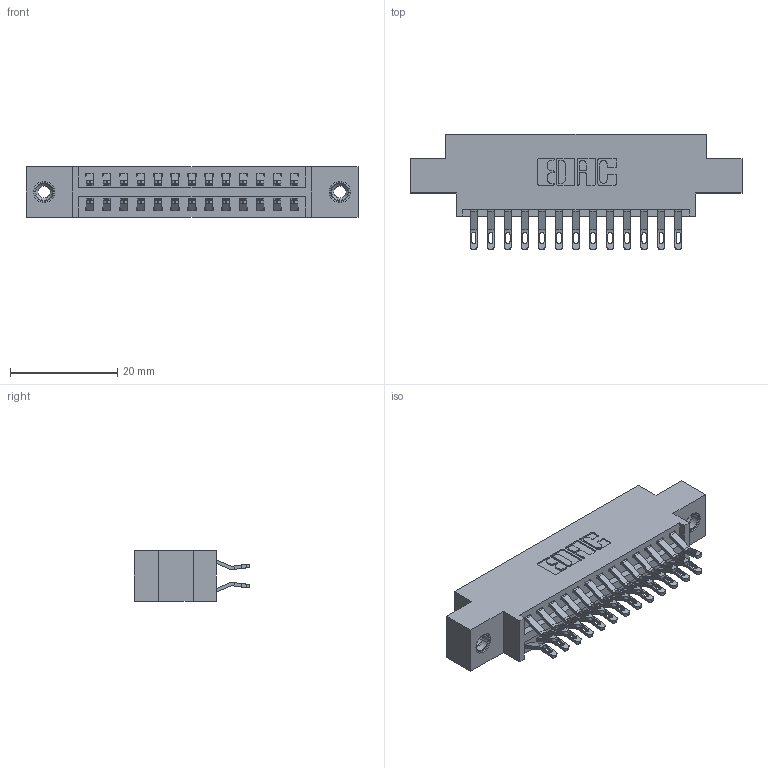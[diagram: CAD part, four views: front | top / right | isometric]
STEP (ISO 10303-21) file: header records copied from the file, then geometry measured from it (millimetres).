
FILE_DESCRIPTION (( 'STEP AP203' ), '1' );
FILE_NAME ('396-026-555-808.STEP', '2018-09-05T00:37:01', ( '' ), ( '' ), 'SwSTEP 2.0', 'SolidWorks 2016', '' );
FILE_SCHEMA (( 'CONFIG_CONTROL_DESIGN' ));
Length unit declared in the file: inch
Products named in the file (4): 346 Part_0.170 Offset - 0.156 Dia-TI; 345-292-001_555 Tail; 345-250-001_345-250-003-102; 396-026-555-808
Assembly tree (29 placements, depth 2):
  396-026-555-808
    346 Part_0.170 Offset - 0.156 Dia-TI
    345-292-001_555 Tail  x26
    345-250-001_345-250-003-102  x2
Bounding box: 61.85 x 21.46 x 9.4 mm (x, y, z)
Volume: 5720.1 mm3; surface area: 7875.3 mm2
Topology: 29 solids, 29 shells, 1694 faces, 5235 edges, 3482 vertices
Faces by surface type: plane 970, cylinder 708, cone 12, torus 4
Entity records: 14032 total; most frequent: CARTESIAN_POINT 2373, ORIENTED_EDGE 2270, DIRECTION 2137, EDGE_CURVE 1135, LINE 911, VECTOR 911, VERTEX_POINT 752, AXIS2_PLACEMENT_3D 613
